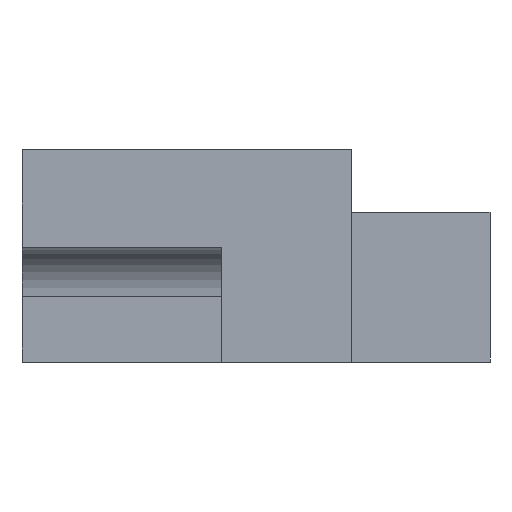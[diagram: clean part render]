
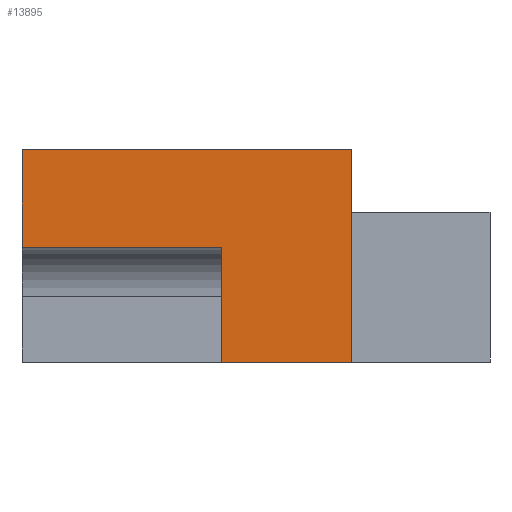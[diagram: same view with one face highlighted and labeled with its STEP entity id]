
A CAD part, left-side view. The second image highlights one B-rep face of the part: STEP entity #13895.
In plain terms, the highlighted planar face has unit normal (-1, 0, 0).
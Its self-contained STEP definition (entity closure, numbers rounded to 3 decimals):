
#344 = VERTEX_POINT ( 'NONE', #12783 ) ;
#517 = LINE ( 'NONE', #659, #15261 ) ;
#577 = DIRECTION ( 'NONE',  ( 0., 0., 1. ) ) ;
#659 = CARTESIAN_POINT ( 'NONE',  ( 0., 0., 0. ) ) ;
#1218 = VECTOR ( 'NONE', #15280, 1000. ) ;
#1720 = VERTEX_POINT ( 'NONE', #8273 ) ;
#2464 = CARTESIAN_POINT ( 'NONE',  ( 0., 8.255, -13.487 ) ) ;
#2590 = ORIENTED_EDGE ( 'NONE', *, *, #21545, .F. ) ;
#4436 = ORIENTED_EDGE ( 'NONE', *, *, #11462, .F. ) ;
#5404 = CARTESIAN_POINT ( 'NONE',  ( 0., 0., 0. ) ) ;
#5715 = CARTESIAN_POINT ( 'NONE',  ( 0., -8.814, -13.487 ) ) ;
#6629 = EDGE_CURVE ( 'NONE', #11710, #16234, #12723, .T. ) ;
#6927 = EDGE_CURVE ( 'NONE', #8287, #11710, #517, .T. ) ;
#7452 = DIRECTION ( 'NONE',  ( 1., 0., 0. ) ) ;
#7874 = CARTESIAN_POINT ( 'NONE',  ( 0., 8.255, -6.172 ) ) ;
#7960 = CARTESIAN_POINT ( 'NONE',  ( 0., 0., 0. ) ) ;
#8273 = CARTESIAN_POINT ( 'NONE',  ( 0., 20.955, -6.172 ) ) ;
#8279 = EDGE_LOOP ( 'NONE', ( #23915, #22991, #18916, #2590, #4436, #9080 ) ) ;
#8287 = VERTEX_POINT ( 'NONE', #7960 ) ;
#8862 = LINE ( 'NONE', #2464, #26085 ) ;
#9080 = ORIENTED_EDGE ( 'NONE', *, *, #13186, .F. ) ;
#9420 = VERTEX_POINT ( 'NONE', #10316 ) ;
#10316 = CARTESIAN_POINT ( 'NONE',  ( 0., 8.255, -6.172 ) ) ;
#11462 = EDGE_CURVE ( 'NONE', #9420, #1720, #18846, .T. ) ;
#11710 = VERTEX_POINT ( 'NONE', #22008 ) ;
#12002 = DIRECTION ( 'NONE',  ( 0., -1., 0. ) ) ;
#12723 = LINE ( 'NONE', #5715, #22918 ) ;
#12783 = CARTESIAN_POINT ( 'NONE',  ( 0., 20.955, 0. ) ) ;
#13186 = EDGE_CURVE ( 'NONE', #16234, #9420, #8862, .T. ) ;
#13327 = VECTOR ( 'NONE', #12002, 1000. ) ;
#13889 = AXIS2_PLACEMENT_3D ( 'NONE', #5404, #7452, #21703 ) ;
#13895 = ADVANCED_FACE ( 'NONE', ( #17445 ), #17618, .F. ) ;
#15261 = VECTOR ( 'NONE', #25042, 1000. ) ;
#15280 = DIRECTION ( 'NONE',  ( 0., 0., 1. ) ) ;
#15895 = LINE ( 'NONE', #18419, #13327 ) ;
#16234 = VERTEX_POINT ( 'NONE', #23995 ) ;
#17445 = FACE_OUTER_BOUND ( 'NONE', #8279, .T. ) ;
#17618 = PLANE ( 'NONE',  #13889 ) ;
#18419 = CARTESIAN_POINT ( 'NONE',  ( 0., 11.506, 0. ) ) ;
#18846 = LINE ( 'NONE', #7874, #23321 ) ;
#18916 = ORIENTED_EDGE ( 'NONE', *, *, #22453, .F. ) ;
#19109 = LINE ( 'NONE', #25351, #1218 ) ;
#19796 = DIRECTION ( 'NONE',  ( 0., 1., 0. ) ) ;
#21545 = EDGE_CURVE ( 'NONE', #1720, #344, #19109, .T. ) ;
#21703 = DIRECTION ( 'NONE',  ( 0., 0., -1. ) ) ;
#22008 = CARTESIAN_POINT ( 'NONE',  ( 0., 0., -13.487 ) ) ;
#22453 = EDGE_CURVE ( 'NONE', #344, #8287, #15895, .T. ) ;
#22918 = VECTOR ( 'NONE', #19796, 1000. ) ;
#22991 = ORIENTED_EDGE ( 'NONE', *, *, #6927, .F. ) ;
#23321 = VECTOR ( 'NONE', #26249, 1000. ) ;
#23915 = ORIENTED_EDGE ( 'NONE', *, *, #6629, .F. ) ;
#23995 = CARTESIAN_POINT ( 'NONE',  ( 0., 8.255, -13.487 ) ) ;
#25042 = DIRECTION ( 'NONE',  ( 0., 0., -1. ) ) ;
#25351 = CARTESIAN_POINT ( 'NONE',  ( 0., 20.955, -13.487 ) ) ;
#26085 = VECTOR ( 'NONE', #577, 1000. ) ;
#26249 = DIRECTION ( 'NONE',  ( 0., 1., 0. ) ) ;
